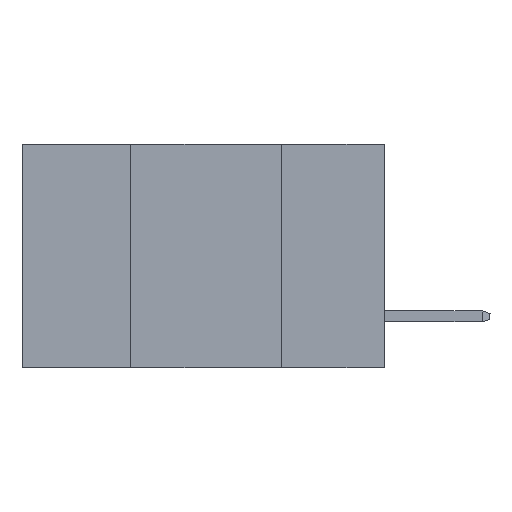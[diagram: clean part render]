
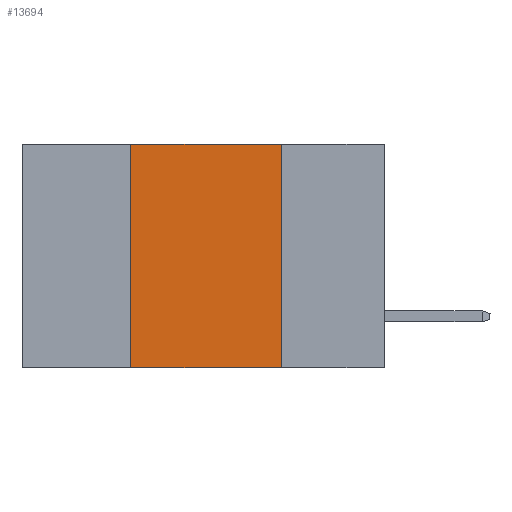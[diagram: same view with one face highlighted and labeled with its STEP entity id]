
A CAD part, left-side view. The second image highlights one B-rep face of the part: STEP entity #13694.
In plain terms, the highlighted planar face has unit normal (-1, 0, 0).
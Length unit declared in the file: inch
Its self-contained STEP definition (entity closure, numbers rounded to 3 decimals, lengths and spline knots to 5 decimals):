
#77 = CARTESIAN_POINT ( 'NONE',  ( 0., 0.6, -0.37 ) ) ;
#773 = ORIENTED_EDGE ( 'NONE', *, *, #13120, .F. ) ;
#809 = CARTESIAN_POINT ( 'NONE',  ( 0., 0.42, 0. ) ) ;
#1870 = PLANE ( 'NONE',  #13453 ) ;
#5243 = LINE ( 'NONE', #14793, #15936 ) ;
#6116 = CARTESIAN_POINT ( 'NONE',  ( 0., 0.6, 0. ) ) ;
#7165 = LINE ( 'NONE', #21892, #15402 ) ;
#7790 = VECTOR ( 'NONE', #20431, 39.37008 ) ;
#7841 = CARTESIAN_POINT ( 'NONE',  ( 0., 0.42, -0.37 ) ) ;
#9340 = DIRECTION ( 'NONE',  ( 0., 0., -1. ) ) ;
#10492 = DIRECTION ( 'NONE',  ( 0., 0., -1. ) ) ;
#11363 = ORIENTED_EDGE ( 'NONE', *, *, #22374, .F. ) ;
#13065 = ORIENTED_EDGE ( 'NONE', *, *, #20021, .F. ) ;
#13120 = EDGE_CURVE ( 'NONE', #14760, #21220, #7165, .T. ) ;
#13453 = AXIS2_PLACEMENT_3D ( 'NONE', #15236, #22209, #9340 ) ;
#13694 = ADVANCED_FACE ( 'NONE', ( #18549 ), #1870, .F. ) ;
#14760 = VERTEX_POINT ( 'NONE', #19925 ) ;
#14793 = CARTESIAN_POINT ( 'NONE',  ( 0., 0.42, -0.37 ) ) ;
#15236 = CARTESIAN_POINT ( 'NONE',  ( 0., 0.6, 0. ) ) ;
#15402 = VECTOR ( 'NONE', #10492, 39.37008 ) ;
#15716 = ORIENTED_EDGE ( 'NONE', *, *, #24082, .T. ) ;
#15936 = VECTOR ( 'NONE', #22266, 39.37008 ) ;
#17821 = CARTESIAN_POINT ( 'NONE',  ( 0., 0.17, -0.37 ) ) ;
#18549 = FACE_OUTER_BOUND ( 'NONE', #22234, .T. ) ;
#19925 = CARTESIAN_POINT ( 'NONE',  ( 0., 0.17, 0. ) ) ;
#20021 = EDGE_CURVE ( 'NONE', #21947, #14760, #22899, .T. ) ;
#20431 = DIRECTION ( 'NONE',  ( 0., -1., 0. ) ) ;
#21220 = VERTEX_POINT ( 'NONE', #17821 ) ;
#21892 = CARTESIAN_POINT ( 'NONE',  ( 0., 0.17, -0.37 ) ) ;
#21947 = VERTEX_POINT ( 'NONE', #809 ) ;
#22130 = LINE ( 'NONE', #77, #7790 ) ;
#22209 = DIRECTION ( 'NONE',  ( 1., 0., 0. ) ) ;
#22234 = EDGE_LOOP ( 'NONE', ( #773, #13065, #11363, #15716 ) ) ;
#22266 = DIRECTION ( 'NONE',  ( 0., 0., 1. ) ) ;
#22374 = EDGE_CURVE ( 'NONE', #23172, #21947, #5243, .T. ) ;
#22899 = LINE ( 'NONE', #6116, #23682 ) ;
#23172 = VERTEX_POINT ( 'NONE', #7841 ) ;
#23366 = DIRECTION ( 'NONE',  ( 0., -1., 0. ) ) ;
#23682 = VECTOR ( 'NONE', #23366, 39.37008 ) ;
#24082 = EDGE_CURVE ( 'NONE', #23172, #21220, #22130, .T. ) ;
